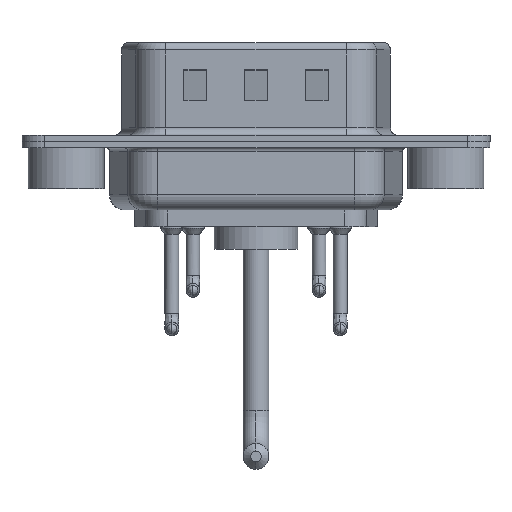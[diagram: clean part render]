
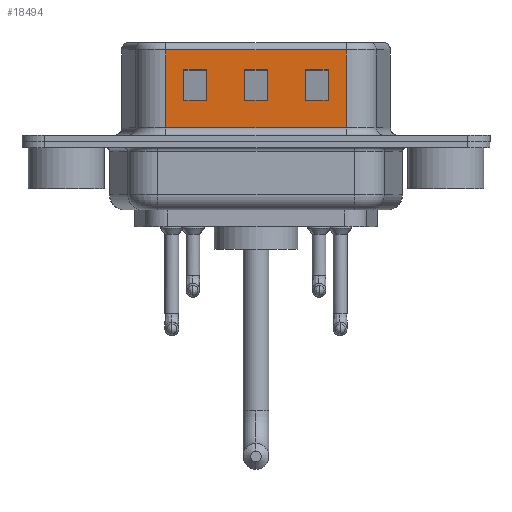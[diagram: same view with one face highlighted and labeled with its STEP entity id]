
A CAD part, front view. The second image highlights one B-rep face of the part: STEP entity #18494.
In plain terms, the highlighted planar face has unit normal (0, -1, 0).
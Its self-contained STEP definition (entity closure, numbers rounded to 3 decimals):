
#129 = ORIENTED_EDGE ( 'NONE', *, *, #3381, .T. ) ;
#221 = VECTOR ( 'NONE', #17430, 1000. ) ;
#326 = ORIENTED_EDGE ( 'NONE', *, *, #3392, .T. ) ;
#496 = DIRECTION ( 'NONE',  ( 0., 0., 1. ) ) ;
#574 = CARTESIAN_POINT ( 'NONE',  ( 17.25, -4.55, 2.705 ) ) ;
#592 = LINE ( 'NONE', #5000, #1334 ) ;
#673 = CARTESIAN_POINT ( 'NONE',  ( 15.75, -4.55, 4.705 ) ) ;
#739 = CARTESIAN_POINT ( 'NONE',  ( 11.75, -4.55, 4.705 ) ) ;
#936 = LINE ( 'NONE', #17605, #16125 ) ;
#943 = EDGE_CURVE ( 'NONE', #13478, #5731, #11524, .T. ) ;
#978 = VECTOR ( 'NONE', #19343, 1000. ) ;
#1180 = CARTESIAN_POINT ( 'NONE',  ( 18.451, -4.55, 6.02 ) ) ;
#1334 = VECTOR ( 'NONE', #496, 1000. ) ;
#1408 = EDGE_LOOP ( 'NONE', ( #9732, #6272, #3024, #16135 ) ) ;
#1605 = FACE_BOUND ( 'NONE', #1408, .T. ) ;
#1618 = EDGE_CURVE ( 'NONE', #10532, #16368, #6184, .T. ) ;
#1694 = CARTESIAN_POINT ( 'NONE',  ( 13.25, -4.55, 4.705 ) ) ;
#2360 = LINE ( 'NONE', #11271, #17356 ) ;
#2415 = VERTEX_POINT ( 'NONE', #7806 ) ;
#2820 = LINE ( 'NONE', #13418, #10341 ) ;
#3024 = ORIENTED_EDGE ( 'NONE', *, *, #10354, .T. ) ;
#3219 = DIRECTION ( 'NONE',  ( 1., 0., 0. ) ) ;
#3381 = EDGE_CURVE ( 'NONE', #2415, #15631, #8324, .T. ) ;
#3392 = EDGE_CURVE ( 'NONE', #5731, #10532, #14302, .T. ) ;
#3555 = ORIENTED_EDGE ( 'NONE', *, *, #4792, .T. ) ;
#3682 = EDGE_LOOP ( 'NONE', ( #11245, #5777, #8988, #19304 ) ) ;
#3786 = ORIENTED_EDGE ( 'NONE', *, *, #14186, .T. ) ;
#3828 = CARTESIAN_POINT ( 'NONE',  ( 17.25, -4.55, 6.52 ) ) ;
#3874 = CARTESIAN_POINT ( 'NONE',  ( 11.75, -4.55, 2.705 ) ) ;
#4231 = VERTEX_POINT ( 'NONE', #15330 ) ;
#4261 = VERTEX_POINT ( 'NONE', #17000 ) ;
#4636 = ORIENTED_EDGE ( 'NONE', *, *, #1618, .T. ) ;
#4792 = EDGE_CURVE ( 'NONE', #16368, #13478, #11481, .T. ) ;
#5000 = CARTESIAN_POINT ( 'NONE',  ( 7.75, -4.55, 6.52 ) ) ;
#5148 = VECTOR ( 'NONE', #3219, 1000. ) ;
#5193 = VERTEX_POINT ( 'NONE', #673 ) ;
#5205 = LINE ( 'NONE', #3828, #7180 ) ;
#5393 = VERTEX_POINT ( 'NONE', #13223 ) ;
#5410 = DIRECTION ( 'NONE',  ( -1., 0., 0. ) ) ;
#5624 = VECTOR ( 'NONE', #6455, 1000. ) ;
#5731 = VERTEX_POINT ( 'NONE', #3874 ) ;
#5777 = ORIENTED_EDGE ( 'NONE', *, *, #17848, .T. ) ;
#5933 = VECTOR ( 'NONE', #6578, 1000. ) ;
#6026 = EDGE_LOOP ( 'NONE', ( #4636, #3555, #15626, #326 ) ) ;
#6184 = LINE ( 'NONE', #16591, #18076 ) ;
#6272 = ORIENTED_EDGE ( 'NONE', *, *, #7037, .T. ) ;
#6455 = DIRECTION ( 'NONE',  ( 0., 0., -1. ) ) ;
#6578 = DIRECTION ( 'NONE',  ( 0., 0., -1. ) ) ;
#6801 = VERTEX_POINT ( 'NONE', #17591 ) ;
#6822 = DIRECTION ( 'NONE',  ( 0., 0., -1. ) ) ;
#6977 = DIRECTION ( 'NONE',  ( 0., 0., -1. ) ) ;
#7037 = EDGE_CURVE ( 'NONE', #15366, #4261, #7391, .T. ) ;
#7180 = VECTOR ( 'NONE', #6977, 1000. ) ;
#7305 = CARTESIAN_POINT ( 'NONE',  ( 6.549, -4.55, 6.02 ) ) ;
#7391 = LINE ( 'NONE', #13375, #978 ) ;
#7394 = CARTESIAN_POINT ( 'NONE',  ( 18.451, -4.55, 6.52 ) ) ;
#7593 = FACE_BOUND ( 'NONE', #6026, .T. ) ;
#7687 = DIRECTION ( 'NONE',  ( -1., 0., 0. ) ) ;
#7806 = CARTESIAN_POINT ( 'NONE',  ( 7.75, -4.55, 4.705 ) ) ;
#8286 = CARTESIAN_POINT ( 'NONE',  ( 7.75, -4.55, 2.705 ) ) ;
#8324 = LINE ( 'NONE', #18612, #8367 ) ;
#8367 = VECTOR ( 'NONE', #18704, 1000. ) ;
#8882 = CARTESIAN_POINT ( 'NONE',  ( 9.25, -4.55, 4.705 ) ) ;
#8893 = VECTOR ( 'NONE', #19385, 1000. ) ;
#8988 = ORIENTED_EDGE ( 'NONE', *, *, #15241, .T. ) ;
#9438 = EDGE_CURVE ( 'NONE', #15631, #5393, #936, .T. ) ;
#9633 = ORIENTED_EDGE ( 'NONE', *, *, #11353, .T. ) ;
#9732 = ORIENTED_EDGE ( 'NONE', *, *, #14991, .T. ) ;
#9876 = VERTEX_POINT ( 'NONE', #12693 ) ;
#10007 = CARTESIAN_POINT ( 'NONE',  ( 13.25, -4.55, 6.52 ) ) ;
#10318 = DIRECTION ( 'NONE',  ( 1., 0., 0. ) ) ;
#10341 = VECTOR ( 'NONE', #16359, 1000. ) ;
#10354 = EDGE_CURVE ( 'NONE', #4261, #5193, #17178, .T. ) ;
#10532 = VERTEX_POINT ( 'NONE', #739 ) ;
#10712 = VERTEX_POINT ( 'NONE', #7305 ) ;
#10977 = LINE ( 'NONE', #15291, #5624 ) ;
#11245 = ORIENTED_EDGE ( 'NONE', *, *, #17054, .F. ) ;
#11271 = CARTESIAN_POINT ( 'NONE',  ( 14.451, -4.55, 2.705 ) ) ;
#11353 = EDGE_CURVE ( 'NONE', #15932, #2415, #592, .T. ) ;
#11370 = DIRECTION ( 'NONE',  ( -1., 0., 0. ) ) ;
#11481 = LINE ( 'NONE', #10007, #5933 ) ;
#11524 = LINE ( 'NONE', #14664, #12781 ) ;
#11855 = EDGE_CURVE ( 'NONE', #9876, #6801, #16661, .T. ) ;
#11973 = DIRECTION ( 'NONE',  ( 1., 0., 0. ) ) ;
#12164 = LINE ( 'NONE', #15115, #12805 ) ;
#12693 = CARTESIAN_POINT ( 'NONE',  ( 6.549, -4.55, 0.9 ) ) ;
#12770 = VECTOR ( 'NONE', #5410, 1000. ) ;
#12781 = VECTOR ( 'NONE', #17503, 1000. ) ;
#12805 = VECTOR ( 'NONE', #11973, 1000. ) ;
#12933 = CARTESIAN_POINT ( 'NONE',  ( 11.75, -4.55, 6.52 ) ) ;
#13223 = CARTESIAN_POINT ( 'NONE',  ( 9.25, -4.55, 2.705 ) ) ;
#13375 = CARTESIAN_POINT ( 'NONE',  ( 22.451, -4.55, 2.705 ) ) ;
#13416 = CARTESIAN_POINT ( 'NONE',  ( 15.75, -4.55, 6.52 ) ) ;
#13418 = CARTESIAN_POINT ( 'NONE',  ( 18.451, -4.55, 6.52 ) ) ;
#13478 = VERTEX_POINT ( 'NONE', #16603 ) ;
#13533 = CARTESIAN_POINT ( 'NONE',  ( 18.451, -4.55, 0.9 ) ) ;
#13573 = FACE_OUTER_BOUND ( 'NONE', #3682, .T. ) ;
#14186 = EDGE_CURVE ( 'NONE', #5393, #15932, #2360, .T. ) ;
#14302 = LINE ( 'NONE', #12933, #221 ) ;
#14626 = LINE ( 'NONE', #1180, #12770 ) ;
#14664 = CARTESIAN_POINT ( 'NONE',  ( 18.451, -4.55, 2.705 ) ) ;
#14846 = PLANE ( 'NONE',  #18099 ) ;
#14991 = EDGE_CURVE ( 'NONE', #19271, #15366, #5205, .T. ) ;
#15047 = FACE_BOUND ( 'NONE', #18760, .T. ) ;
#15115 = CARTESIAN_POINT ( 'NONE',  ( 22.451, -4.55, 4.705 ) ) ;
#15241 = EDGE_CURVE ( 'NONE', #10712, #9876, #10977, .T. ) ;
#15291 = CARTESIAN_POINT ( 'NONE',  ( 6.549, -4.55, 6.52 ) ) ;
#15330 = CARTESIAN_POINT ( 'NONE',  ( 18.451, -4.55, 6.02 ) ) ;
#15366 = VERTEX_POINT ( 'NONE', #574 ) ;
#15626 = ORIENTED_EDGE ( 'NONE', *, *, #943, .T. ) ;
#15631 = VERTEX_POINT ( 'NONE', #8882 ) ;
#15932 = VERTEX_POINT ( 'NONE', #8286 ) ;
#16125 = VECTOR ( 'NONE', #6822, 1000. ) ;
#16135 = ORIENTED_EDGE ( 'NONE', *, *, #18896, .T. ) ;
#16359 = DIRECTION ( 'NONE',  ( 0., 0., -1. ) ) ;
#16368 = VERTEX_POINT ( 'NONE', #1694 ) ;
#16591 = CARTESIAN_POINT ( 'NONE',  ( 18.451, -4.55, 4.705 ) ) ;
#16603 = CARTESIAN_POINT ( 'NONE',  ( 13.25, -4.55, 2.705 ) ) ;
#16661 = LINE ( 'NONE', #13533, #5148 ) ;
#17000 = CARTESIAN_POINT ( 'NONE',  ( 15.75, -4.55, 2.705 ) ) ;
#17054 = EDGE_CURVE ( 'NONE', #4231, #6801, #2820, .T. ) ;
#17178 = LINE ( 'NONE', #13416, #8893 ) ;
#17356 = VECTOR ( 'NONE', #11370, 1000. ) ;
#17430 = DIRECTION ( 'NONE',  ( 0., 0., 1. ) ) ;
#17503 = DIRECTION ( 'NONE',  ( -1., 0., 0. ) ) ;
#17591 = CARTESIAN_POINT ( 'NONE',  ( 18.451, -4.55, 0.9 ) ) ;
#17605 = CARTESIAN_POINT ( 'NONE',  ( 9.25, -4.55, 6.52 ) ) ;
#17848 = EDGE_CURVE ( 'NONE', #4231, #10712, #14626, .T. ) ;
#17934 = CARTESIAN_POINT ( 'NONE',  ( 17.25, -4.55, 4.705 ) ) ;
#18076 = VECTOR ( 'NONE', #10318, 1000. ) ;
#18099 = AXIS2_PLACEMENT_3D ( 'NONE', #7394, #19348, #7687 ) ;
#18494 = ADVANCED_FACE ( 'NONE', ( #15047, #1605, #7593, #13573 ), #14846, .F. ) ;
#18612 = CARTESIAN_POINT ( 'NONE',  ( 14.451, -4.55, 4.705 ) ) ;
#18704 = DIRECTION ( 'NONE',  ( 1., 0., 0. ) ) ;
#18758 = ORIENTED_EDGE ( 'NONE', *, *, #9438, .T. ) ;
#18760 = EDGE_LOOP ( 'NONE', ( #18758, #3786, #9633, #129 ) ) ;
#18896 = EDGE_CURVE ( 'NONE', #5193, #19271, #12164, .T. ) ;
#19271 = VERTEX_POINT ( 'NONE', #17934 ) ;
#19304 = ORIENTED_EDGE ( 'NONE', *, *, #11855, .T. ) ;
#19343 = DIRECTION ( 'NONE',  ( -1., 0., 0. ) ) ;
#19348 = DIRECTION ( 'NONE',  ( 0., 1., 0. ) ) ;
#19385 = DIRECTION ( 'NONE',  ( 0., 0., 1. ) ) ;
